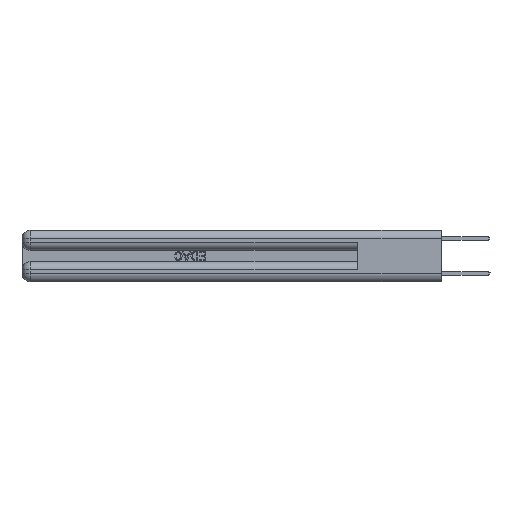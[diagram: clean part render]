
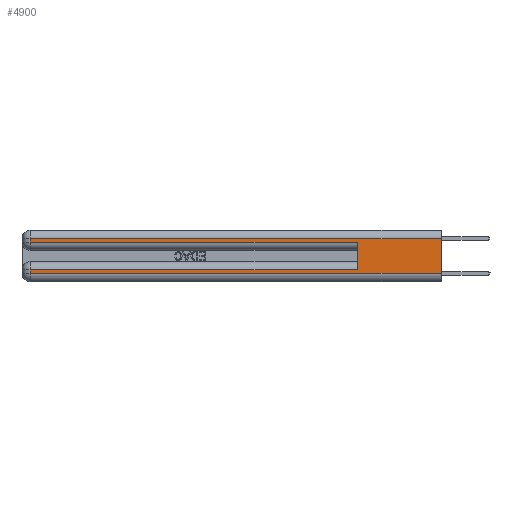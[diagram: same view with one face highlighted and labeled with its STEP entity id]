
A CAD part, left-side view. The second image highlights one B-rep face of the part: STEP entity #4900.
In plain terms, the highlighted planar face has unit normal (-1, 0, 0).
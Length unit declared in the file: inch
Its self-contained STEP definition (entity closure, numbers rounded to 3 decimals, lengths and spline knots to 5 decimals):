
#21 = LINE ( 'NONE', #31209, #24242 ) ;
#220 = EDGE_CURVE ( 'NONE', #17919, #18934, #13119, .T. ) ;
#333 = LINE ( 'NONE', #4336, #16718 ) ;
#500 = VECTOR ( 'NONE', #22743, 39.37008 ) ;
#618 = EDGE_CURVE ( 'NONE', #11972, #16497, #24782, .T. ) ;
#3252 = EDGE_CURVE ( 'NONE', #15185, #7641, #21, .T. ) ;
#3600 = CARTESIAN_POINT ( 'NONE',  ( 0., 0., 0.31 ) ) ;
#4336 = CARTESIAN_POINT ( 'NONE',  ( 0., 0., 0.285 ) ) ;
#4900 = ADVANCED_FACE ( 'NONE', ( #9820 ), #7548, .F. ) ;
#5330 = CARTESIAN_POINT ( 'NONE',  ( 0., 0., 0.06 ) ) ;
#7067 = DIRECTION ( 'NONE',  ( 0., -1., 0. ) ) ;
#7338 = CARTESIAN_POINT ( 'NONE',  ( 0., 2.94, 0.06 ) ) ;
#7548 = PLANE ( 'NONE',  #12684 ) ;
#7641 = VERTEX_POINT ( 'NONE', #15886 ) ;
#7953 = ORIENTED_EDGE ( 'NONE', *, *, #220, .F. ) ;
#8046 = ORIENTED_EDGE ( 'NONE', *, *, #3252, .F. ) ;
#8603 = CARTESIAN_POINT ( 'NONE',  ( 0., 2.94, 0.31 ) ) ;
#8614 = VERTEX_POINT ( 'NONE', #18438 ) ;
#9820 = FACE_OUTER_BOUND ( 'NONE', #11493, .T. ) ;
#10451 = EDGE_CURVE ( 'NONE', #8614, #23216, #14889, .T. ) ;
#11341 = VECTOR ( 'NONE', #25494, 39.37008 ) ;
#11493 = EDGE_LOOP ( 'NONE', ( #7953, #20581, #23752, #25708, #8046, #33534, #22324, #31170 ) ) ;
#11722 = CARTESIAN_POINT ( 'NONE',  ( 0., 0., 0.31 ) ) ;
#11972 = VERTEX_POINT ( 'NONE', #8603 ) ;
#12353 = CARTESIAN_POINT ( 'NONE',  ( 0., 2.94, 0.37 ) ) ;
#12684 = AXIS2_PLACEMENT_3D ( 'NONE', #29768, #32678, #21348 ) ;
#13119 = LINE ( 'NONE', #27446, #18311 ) ;
#13585 = EDGE_CURVE ( 'NONE', #17919, #11972, #15903, .T. ) ;
#14889 = LINE ( 'NONE', #32147, #30855 ) ;
#15185 = VERTEX_POINT ( 'NONE', #24417 ) ;
#15348 = EDGE_CURVE ( 'NONE', #16497, #7641, #333, .T. ) ;
#15886 = CARTESIAN_POINT ( 'NONE',  ( 0., 0.6, 0.285 ) ) ;
#15903 = LINE ( 'NONE', #11722, #30573 ) ;
#16412 = DIRECTION ( 'NONE',  ( 0., 0., -1. ) ) ;
#16497 = VERTEX_POINT ( 'NONE', #25837 ) ;
#16718 = VECTOR ( 'NONE', #7067, 39.37008 ) ;
#17038 = CARTESIAN_POINT ( 'NONE',  ( 0., 0., 0.06 ) ) ;
#17919 = VERTEX_POINT ( 'NONE', #3600 ) ;
#18311 = VECTOR ( 'NONE', #16412, 39.37008 ) ;
#18438 = CARTESIAN_POINT ( 'NONE',  ( 0., 2.94, 0.085 ) ) ;
#18934 = VERTEX_POINT ( 'NONE', #5330 ) ;
#19573 = VECTOR ( 'NONE', #21031, 39.37008 ) ;
#20581 = ORIENTED_EDGE ( 'NONE', *, *, #13585, .T. ) ;
#21031 = DIRECTION ( 'NONE',  ( 0., 0., -1. ) ) ;
#21348 = DIRECTION ( 'NONE',  ( 0., 0., -1. ) ) ;
#22324 = ORIENTED_EDGE ( 'NONE', *, *, #10451, .T. ) ;
#22743 = DIRECTION ( 'NONE',  ( 0., -1., 0. ) ) ;
#23216 = VERTEX_POINT ( 'NONE', #7338 ) ;
#23752 = ORIENTED_EDGE ( 'NONE', *, *, #618, .T. ) ;
#24242 = VECTOR ( 'NONE', #30969, 39.37008 ) ;
#24250 = LINE ( 'NONE', #17038, #500 ) ;
#24360 = DIRECTION ( 'NONE',  ( 0., 0., -1. ) ) ;
#24417 = CARTESIAN_POINT ( 'NONE',  ( 0., 0.6, 0.085 ) ) ;
#24650 = EDGE_CURVE ( 'NONE', #23216, #18934, #24250, .T. ) ;
#24782 = LINE ( 'NONE', #12353, #19573 ) ;
#25494 = DIRECTION ( 'NONE',  ( 0., 1., 0. ) ) ;
#25708 = ORIENTED_EDGE ( 'NONE', *, *, #15348, .T. ) ;
#25837 = CARTESIAN_POINT ( 'NONE',  ( 0., 2.94, 0.285 ) ) ;
#27446 = CARTESIAN_POINT ( 'NONE',  ( 0., 0., 0.37 ) ) ;
#27807 = LINE ( 'NONE', #34376, #11341 ) ;
#29768 = CARTESIAN_POINT ( 'NONE',  ( 0., 0., 0.37 ) ) ;
#30573 = VECTOR ( 'NONE', #30996, 39.37008 ) ;
#30855 = VECTOR ( 'NONE', #24360, 39.37008 ) ;
#30969 = DIRECTION ( 'NONE',  ( 0., 0., 1. ) ) ;
#30996 = DIRECTION ( 'NONE',  ( 0., 1., 0. ) ) ;
#31170 = ORIENTED_EDGE ( 'NONE', *, *, #24650, .T. ) ;
#31209 = CARTESIAN_POINT ( 'NONE',  ( 0., 0.6, 0.145 ) ) ;
#32147 = CARTESIAN_POINT ( 'NONE',  ( 0., 2.94, 0.37 ) ) ;
#32678 = DIRECTION ( 'NONE',  ( 1., 0., 0. ) ) ;
#33534 = ORIENTED_EDGE ( 'NONE', *, *, #33709, .T. ) ;
#33709 = EDGE_CURVE ( 'NONE', #15185, #8614, #27807, .T. ) ;
#34376 = CARTESIAN_POINT ( 'NONE',  ( 0., 0., 0.085 ) ) ;
